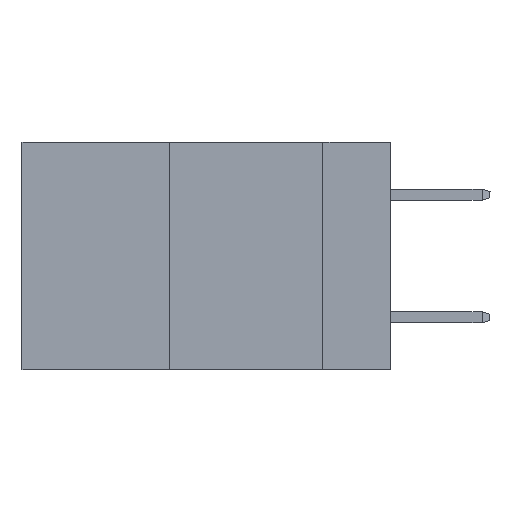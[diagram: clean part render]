
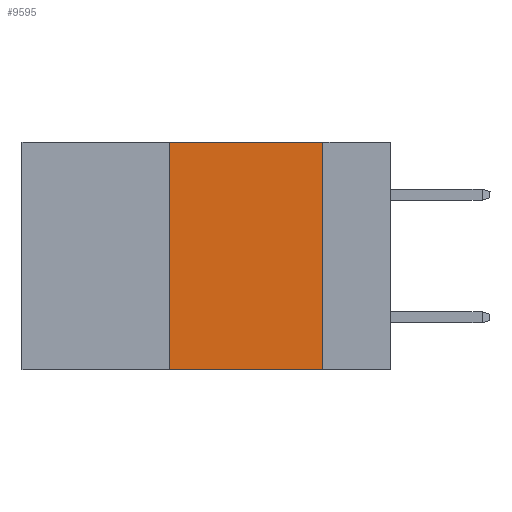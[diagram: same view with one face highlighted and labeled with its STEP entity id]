
A CAD part, left-side view. The second image highlights one B-rep face of the part: STEP entity #9595.
In plain terms, the highlighted planar face has unit normal (-1, 0, 0).
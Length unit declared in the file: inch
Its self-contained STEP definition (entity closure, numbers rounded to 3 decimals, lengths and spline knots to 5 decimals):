
#293 = EDGE_CURVE ( 'NONE', #23695, #6949, #2296, .T. ) ;
#532 = FACE_OUTER_BOUND ( 'NONE', #7134, .T. ) ;
#1460 = ORIENTED_EDGE ( 'NONE', *, *, #19980, .F. ) ;
#1485 = VECTOR ( 'NONE', #8778, 39.37008 ) ;
#1612 = AXIS2_PLACEMENT_3D ( 'NONE', #1709, #3765, #17726 ) ;
#1709 = CARTESIAN_POINT ( 'NONE',  ( 0., 0.6, 0. ) ) ;
#2296 = LINE ( 'NONE', #25213, #21056 ) ;
#2329 = CARTESIAN_POINT ( 'NONE',  ( 0., 0.6, 0. ) ) ;
#2417 = DIRECTION ( 'NONE',  ( 0., -1., 0. ) ) ;
#2426 = VERTEX_POINT ( 'NONE', #24303 ) ;
#3765 = DIRECTION ( 'NONE',  ( 1., 0., 0. ) ) ;
#3943 = EDGE_CURVE ( 'NONE', #23695, #2426, #16861, .T. ) ;
#4030 = ORIENTED_EDGE ( 'NONE', *, *, #3943, .F. ) ;
#6949 = VERTEX_POINT ( 'NONE', #16969 ) ;
#7093 = VECTOR ( 'NONE', #11661, 39.37008 ) ;
#7134 = EDGE_LOOP ( 'NONE', ( #1460, #8128, #4030, #22436 ) ) ;
#7726 = CARTESIAN_POINT ( 'NONE',  ( 0., 0.11, 0. ) ) ;
#8128 = ORIENTED_EDGE ( 'NONE', *, *, #17595, .F. ) ;
#8778 = DIRECTION ( 'NONE',  ( 0., 0., 1. ) ) ;
#9595 = ADVANCED_FACE ( 'NONE', ( #532 ), #13782, .F. ) ;
#10970 = VECTOR ( 'NONE', #2417, 39.37008 ) ;
#11661 = DIRECTION ( 'NONE',  ( 0., 0., -1. ) ) ;
#13782 = PLANE ( 'NONE',  #1612 ) ;
#15353 = DIRECTION ( 'NONE',  ( 0., -1., 0. ) ) ;
#16265 = LINE ( 'NONE', #2329, #10970 ) ;
#16506 = CARTESIAN_POINT ( 'NONE',  ( 0., 0.36, -0.37 ) ) ;
#16861 = LINE ( 'NONE', #18671, #1485 ) ;
#16969 = CARTESIAN_POINT ( 'NONE',  ( 0., 0.11, -0.37 ) ) ;
#17595 = EDGE_CURVE ( 'NONE', #2426, #19984, #16265, .T. ) ;
#17726 = DIRECTION ( 'NONE',  ( 0., 0., -1. ) ) ;
#18671 = CARTESIAN_POINT ( 'NONE',  ( 0., 0.36, 0. ) ) ;
#19980 = EDGE_CURVE ( 'NONE', #19984, #6949, #22350, .T. ) ;
#19984 = VERTEX_POINT ( 'NONE', #23641 ) ;
#21056 = VECTOR ( 'NONE', #15353, 39.37008 ) ;
#22350 = LINE ( 'NONE', #7726, #7093 ) ;
#22436 = ORIENTED_EDGE ( 'NONE', *, *, #293, .T. ) ;
#23641 = CARTESIAN_POINT ( 'NONE',  ( 0., 0.11, 0. ) ) ;
#23695 = VERTEX_POINT ( 'NONE', #16506 ) ;
#24303 = CARTESIAN_POINT ( 'NONE',  ( 0., 0.36, 0. ) ) ;
#25213 = CARTESIAN_POINT ( 'NONE',  ( 0., 0.6, -0.37 ) ) ;
